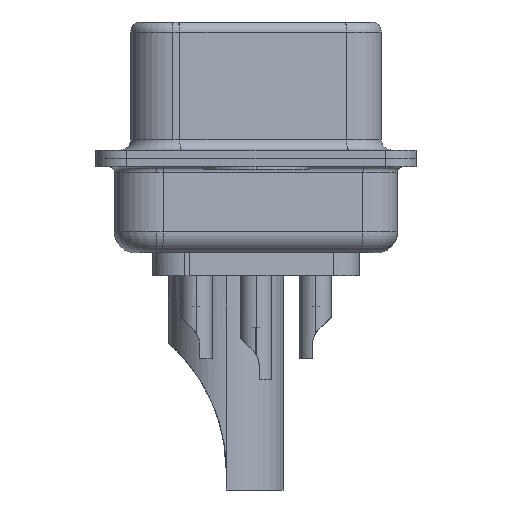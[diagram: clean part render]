
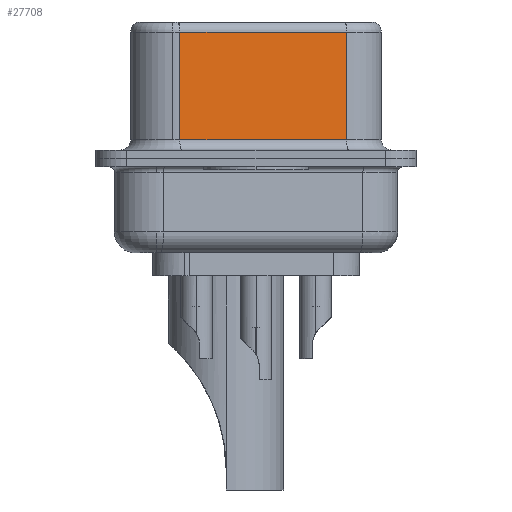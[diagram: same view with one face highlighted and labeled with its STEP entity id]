
A CAD part, left-side view. The second image highlights one B-rep face of the part: STEP entity #27708.
In plain terms, the highlighted planar face has unit normal (-0.985, -0.174, 0).
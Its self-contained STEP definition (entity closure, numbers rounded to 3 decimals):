
#103 = VERTEX_POINT ( 'NONE', #695 ) ;
#574 = ORIENTED_EDGE ( 'NONE', *, *, #14594, .T. ) ;
#695 = CARTESIAN_POINT ( 'NONE',  ( 5.132, -4.322, 6.02 ) ) ;
#1638 = CARTESIAN_POINT ( 'NONE',  ( 5.132, -4.322, 0.9 ) ) ;
#2032 = VECTOR ( 'NONE', #9081, 1000. ) ;
#2223 = VECTOR ( 'NONE', #16923, 1000. ) ;
#2411 = DIRECTION ( 'NONE',  ( 0., 0., -1. ) ) ;
#3282 = ORIENTED_EDGE ( 'NONE', *, *, #11376, .T. ) ;
#4471 = EDGE_CURVE ( 'NONE', #103, #15656, #10806, .T. ) ;
#4954 = LINE ( 'NONE', #10465, #2223 ) ;
#7424 = VERTEX_POINT ( 'NONE', #15230 ) ;
#7991 = ORIENTED_EDGE ( 'NONE', *, *, #4471, .F. ) ;
#8221 = EDGE_LOOP ( 'NONE', ( #7991, #9684, #574, #3282 ) ) ;
#9081 = DIRECTION ( 'NONE',  ( 0., 0., -1. ) ) ;
#9684 = ORIENTED_EDGE ( 'NONE', *, *, #23198, .T. ) ;
#10465 = CARTESIAN_POINT ( 'NONE',  ( 5.132, -4.322, 0.9 ) ) ;
#10505 = DIRECTION ( 'NONE',  ( 0.985, 0.174, 0. ) ) ;
#10782 = LINE ( 'NONE', #15788, #2032 ) ;
#10806 = LINE ( 'NONE', #24310, #19278 ) ;
#11376 = EDGE_CURVE ( 'NONE', #16948, #15656, #4954, .T. ) ;
#14020 = CARTESIAN_POINT ( 'NONE',  ( 3.73, 3.628, 0.9 ) ) ;
#14515 = LINE ( 'NONE', #25738, #20287 ) ;
#14594 = EDGE_CURVE ( 'NONE', #7424, #16948, #10782, .T. ) ;
#14890 = CARTESIAN_POINT ( 'NONE',  ( 5.132, -4.322, 6.52 ) ) ;
#15230 = CARTESIAN_POINT ( 'NONE',  ( 3.73, 3.628, 6.02 ) ) ;
#15656 = VERTEX_POINT ( 'NONE', #1638 ) ;
#15788 = CARTESIAN_POINT ( 'NONE',  ( 3.73, 3.628, 6.52 ) ) ;
#16923 = DIRECTION ( 'NONE',  ( 0.174, -0.985, 0. ) ) ;
#16948 = VERTEX_POINT ( 'NONE', #14020 ) ;
#18861 = DIRECTION ( 'NONE',  ( -0.174, 0.985, 0. ) ) ;
#19222 = DIRECTION ( 'NONE',  ( -0.174, 0.985, 0. ) ) ;
#19278 = VECTOR ( 'NONE', #2411, 1000. ) ;
#20287 = VECTOR ( 'NONE', #19222, 1000. ) ;
#21734 = FACE_OUTER_BOUND ( 'NONE', #8221, .T. ) ;
#23198 = EDGE_CURVE ( 'NONE', #103, #7424, #14515, .T. ) ;
#23433 = AXIS2_PLACEMENT_3D ( 'NONE', #14890, #10505, #18861 ) ;
#24310 = CARTESIAN_POINT ( 'NONE',  ( 5.132, -4.322, 6.52 ) ) ;
#25374 = PLANE ( 'NONE',  #23433 ) ;
#25738 = CARTESIAN_POINT ( 'NONE',  ( 5.132, -4.322, 6.02 ) ) ;
#27708 = ADVANCED_FACE ( 'NONE', ( #21734 ), #25374, .F. ) ;
